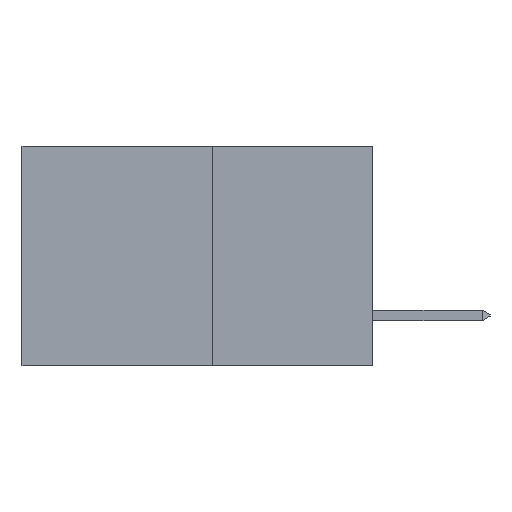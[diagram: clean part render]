
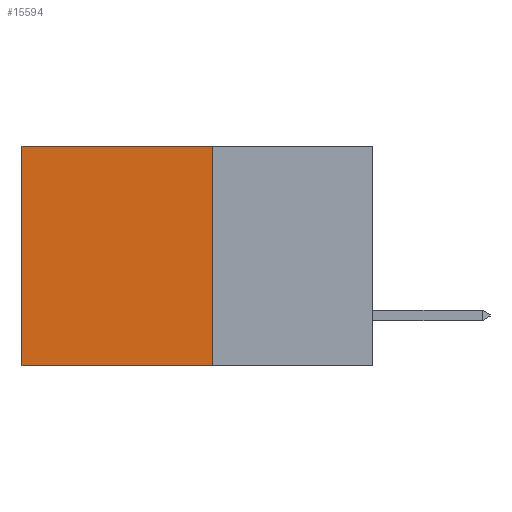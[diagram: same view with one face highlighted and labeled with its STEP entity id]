
A CAD part, left-side view. The second image highlights one B-rep face of the part: STEP entity #15594.
In plain terms, the highlighted planar face has unit normal (-1, 0, 0).
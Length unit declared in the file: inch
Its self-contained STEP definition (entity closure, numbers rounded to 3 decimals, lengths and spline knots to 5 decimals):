
#143 = VECTOR ( 'NONE', #6793, 39.37008 ) ;
#712 = CARTESIAN_POINT ( 'NONE',  ( 0.277, 0.27, 0. ) ) ;
#1078 = VERTEX_POINT ( 'NONE', #712 ) ;
#1534 = CARTESIAN_POINT ( 'NONE',  ( 0.277, 0.59, 0. ) ) ;
#3578 = VERTEX_POINT ( 'NONE', #17851 ) ;
#5021 = CARTESIAN_POINT ( 'NONE',  ( 0.277, 0.59, -0.37 ) ) ;
#5032 = ORIENTED_EDGE ( 'NONE', *, *, #8994, .F. ) ;
#5941 = CARTESIAN_POINT ( 'NONE',  ( 0.277, 0.27, -0.37 ) ) ;
#6793 = DIRECTION ( 'NONE',  ( 0., 0., -1. ) ) ;
#7005 = LINE ( 'NONE', #17709, #11679 ) ;
#7433 = LINE ( 'NONE', #20995, #16172 ) ;
#7477 = PLANE ( 'NONE',  #15580 ) ;
#8473 = ORIENTED_EDGE ( 'NONE', *, *, #14102, .T. ) ;
#8812 = VECTOR ( 'NONE', #11165, 39.37008 ) ;
#8940 = DIRECTION ( 'NONE',  ( 0., 0., -1. ) ) ;
#8994 = EDGE_CURVE ( 'NONE', #3578, #16389, #17506, .T. ) ;
#9197 = DIRECTION ( 'NONE',  ( 1., 0., 0. ) ) ;
#11165 = DIRECTION ( 'NONE',  ( 0., 1., 0. ) ) ;
#11448 = CARTESIAN_POINT ( 'NONE',  ( 0.277, 0.59, -0.37 ) ) ;
#11679 = VECTOR ( 'NONE', #19413, 39.37008 ) ;
#11827 = ORIENTED_EDGE ( 'NONE', *, *, #17582, .F. ) ;
#14102 = EDGE_CURVE ( 'NONE', #14793, #16389, #14146, .T. ) ;
#14146 = LINE ( 'NONE', #5021, #143 ) ;
#14793 = VERTEX_POINT ( 'NONE', #1534 ) ;
#15553 = EDGE_CURVE ( 'NONE', #1078, #14793, #7005, .T. ) ;
#15580 = AXIS2_PLACEMENT_3D ( 'NONE', #17860, #9197, #21236 ) ;
#15594 = ADVANCED_FACE ( 'NONE', ( #19155 ), #7477, .F. ) ;
#16172 = VECTOR ( 'NONE', #8940, 39.37008 ) ;
#16389 = VERTEX_POINT ( 'NONE', #11448 ) ;
#17506 = LINE ( 'NONE', #5941, #8812 ) ;
#17582 = EDGE_CURVE ( 'NONE', #1078, #3578, #7433, .T. ) ;
#17709 = CARTESIAN_POINT ( 'NONE',  ( 0.277, 0.27, 0. ) ) ;
#17851 = CARTESIAN_POINT ( 'NONE',  ( 0.277, 0.27, -0.37 ) ) ;
#17860 = CARTESIAN_POINT ( 'NONE',  ( 0.277, 0.27, -0.37 ) ) ;
#19155 = FACE_OUTER_BOUND ( 'NONE', #20558, .T. ) ;
#19413 = DIRECTION ( 'NONE',  ( 0., 1., 0. ) ) ;
#20558 = EDGE_LOOP ( 'NONE', ( #8473, #5032, #11827, #20881 ) ) ;
#20881 = ORIENTED_EDGE ( 'NONE', *, *, #15553, .T. ) ;
#20995 = CARTESIAN_POINT ( 'NONE',  ( 0.277, 0.27, -0.37 ) ) ;
#21236 = DIRECTION ( 'NONE',  ( 0., 0., -1. ) ) ;
